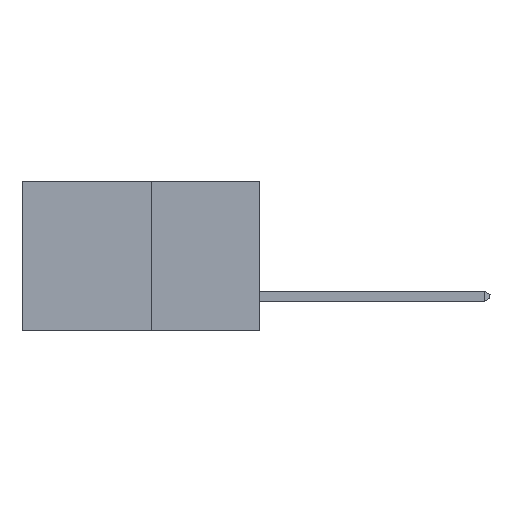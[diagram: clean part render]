
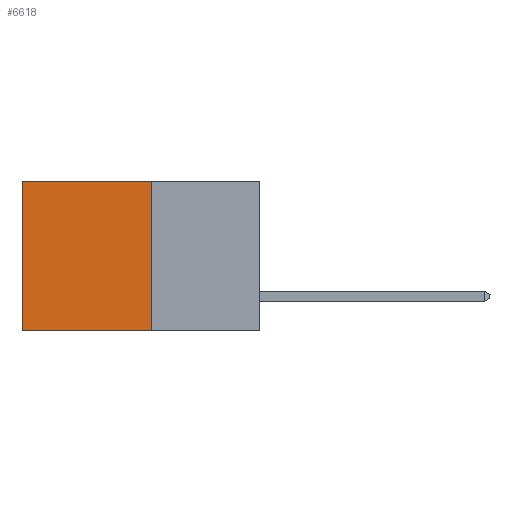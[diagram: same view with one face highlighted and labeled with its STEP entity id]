
A CAD part, left-side view. The second image highlights one B-rep face of the part: STEP entity #6618.
In plain terms, the highlighted planar face has unit normal (-1, 0, 0).
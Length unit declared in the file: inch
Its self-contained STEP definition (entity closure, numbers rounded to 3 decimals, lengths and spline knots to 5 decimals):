
#1 = ORIENTED_EDGE ( 'NONE', *, *, #1493, .T. ) ;
#674 = LINE ( 'NONE', #13691, #10036 ) ;
#1336 = ORIENTED_EDGE ( 'NONE', *, *, #13042, .T. ) ;
#1383 = ORIENTED_EDGE ( 'NONE', *, *, #13606, .F. ) ;
#1493 = EDGE_CURVE ( 'NONE', #11995, #14558, #2851, .T. ) ;
#1497 = ORIENTED_EDGE ( 'NONE', *, *, #9339, .F. ) ;
#1790 = CARTESIAN_POINT ( 'NONE',  ( 0.277, 0.27, -0.37 ) ) ;
#2851 = LINE ( 'NONE', #13068, #10852 ) ;
#3076 = LINE ( 'NONE', #7036, #8835 ) ;
#3553 = VERTEX_POINT ( 'NONE', #5888 ) ;
#3643 = CARTESIAN_POINT ( 'NONE',  ( 0.277, 0.59, 0. ) ) ;
#4269 = DIRECTION ( 'NONE',  ( 0., 0., -1. ) ) ;
#4715 = DIRECTION ( 'NONE',  ( 0., 1., 0. ) ) ;
#5800 = EDGE_LOOP ( 'NONE', ( #1336, #1383, #1497, #1 ) ) ;
#5888 = CARTESIAN_POINT ( 'NONE',  ( 0.277, 0.59, -0.37 ) ) ;
#6044 = AXIS2_PLACEMENT_3D ( 'NONE', #1790, #10969, #4269 ) ;
#6618 = ADVANCED_FACE ( 'NONE', ( #11664 ), #9880, .F. ) ;
#7036 = CARTESIAN_POINT ( 'NONE',  ( 0.277, 0.27, -0.37 ) ) ;
#7295 = CARTESIAN_POINT ( 'NONE',  ( 0.277, 0.27, -0.37 ) ) ;
#8615 = DIRECTION ( 'NONE',  ( 0., 0., -1. ) ) ;
#8835 = VECTOR ( 'NONE', #4715, 39.37008 ) ;
#9339 = EDGE_CURVE ( 'NONE', #11995, #12707, #12442, .T. ) ;
#9558 = VECTOR ( 'NONE', #8615, 39.37008 ) ;
#9880 = PLANE ( 'NONE',  #6044 ) ;
#10036 = VECTOR ( 'NONE', #12666, 39.37008 ) ;
#10852 = VECTOR ( 'NONE', #11200, 39.37008 ) ;
#10969 = DIRECTION ( 'NONE',  ( 1., 0., 0. ) ) ;
#11200 = DIRECTION ( 'NONE',  ( 0., 1., 0. ) ) ;
#11664 = FACE_OUTER_BOUND ( 'NONE', #5800, .T. ) ;
#11848 = CARTESIAN_POINT ( 'NONE',  ( 0.277, 0.27, -0.37 ) ) ;
#11995 = VERTEX_POINT ( 'NONE', #13619 ) ;
#12442 = LINE ( 'NONE', #11848, #9558 ) ;
#12666 = DIRECTION ( 'NONE',  ( 0., 0., -1. ) ) ;
#12707 = VERTEX_POINT ( 'NONE', #7295 ) ;
#13042 = EDGE_CURVE ( 'NONE', #14558, #3553, #674, .T. ) ;
#13068 = CARTESIAN_POINT ( 'NONE',  ( 0.277, 0.27, 0. ) ) ;
#13606 = EDGE_CURVE ( 'NONE', #12707, #3553, #3076, .T. ) ;
#13619 = CARTESIAN_POINT ( 'NONE',  ( 0.277, 0.27, 0. ) ) ;
#13691 = CARTESIAN_POINT ( 'NONE',  ( 0.277, 0.59, -0.37 ) ) ;
#14558 = VERTEX_POINT ( 'NONE', #3643 ) ;
